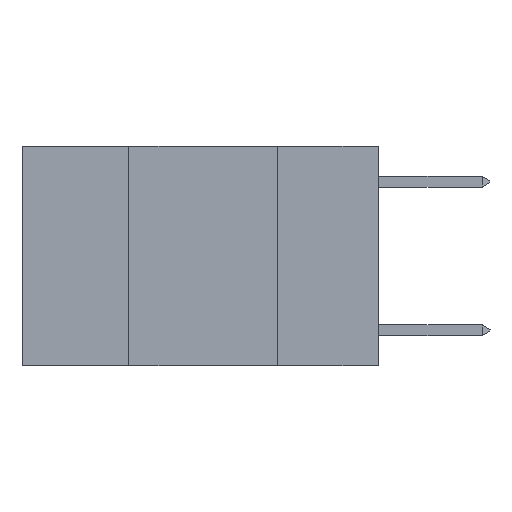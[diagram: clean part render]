
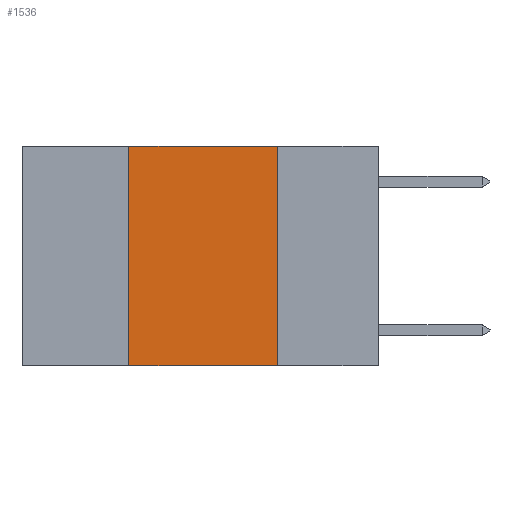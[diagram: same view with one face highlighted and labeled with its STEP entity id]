
A CAD part, left-side view. The second image highlights one B-rep face of the part: STEP entity #1536.
In plain terms, the highlighted planar face has unit normal (-1, 0, 0).
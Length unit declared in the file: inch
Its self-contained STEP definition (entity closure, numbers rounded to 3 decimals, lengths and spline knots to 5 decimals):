
#22 = CARTESIAN_POINT ( 'NONE',  ( 0., 0.17, 0. ) ) ;
#275 = EDGE_CURVE ( 'NONE', #723, #17620, #13090, .T. ) ;
#723 = VERTEX_POINT ( 'NONE', #16171 ) ;
#1536 = ADVANCED_FACE ( 'NONE', ( #12596 ), #6513, .F. ) ;
#1971 = EDGE_LOOP ( 'NONE', ( #5918, #19016, #5933, #5943 ) ) ;
#3739 = CARTESIAN_POINT ( 'NONE',  ( 0., 0.6, -0.37 ) ) ;
#4003 = VECTOR ( 'NONE', #4907, 39.37008 ) ;
#4252 = VERTEX_POINT ( 'NONE', #18036 ) ;
#4571 = CARTESIAN_POINT ( 'NONE',  ( 0., 0.17, -0.37 ) ) ;
#4907 = DIRECTION ( 'NONE',  ( 0., -1., 0. ) ) ;
#5918 = ORIENTED_EDGE ( 'NONE', *, *, #7991, .F. ) ;
#5933 = ORIENTED_EDGE ( 'NONE', *, *, #17792, .F. ) ;
#5943 = ORIENTED_EDGE ( 'NONE', *, *, #275, .T. ) ;
#6513 = PLANE ( 'NONE',  #15474 ) ;
#7655 = EDGE_CURVE ( 'NONE', #4252, #19973, #13603, .T. ) ;
#7675 = DIRECTION ( 'NONE',  ( 0., 0., -1. ) ) ;
#7991 = EDGE_CURVE ( 'NONE', #19973, #17620, #14310, .T. ) ;
#9720 = LINE ( 'NONE', #11394, #17651 ) ;
#11394 = CARTESIAN_POINT ( 'NONE',  ( 0., 0.42, 0. ) ) ;
#12596 = FACE_OUTER_BOUND ( 'NONE', #1971, .T. ) ;
#12691 = DIRECTION ( 'NONE',  ( 1., 0., 0. ) ) ;
#12811 = CARTESIAN_POINT ( 'NONE',  ( 0., 0.17, 0. ) ) ;
#13090 = LINE ( 'NONE', #3739, #4003 ) ;
#13603 = LINE ( 'NONE', #19929, #19804 ) ;
#14310 = LINE ( 'NONE', #22, #16491 ) ;
#15474 = AXIS2_PLACEMENT_3D ( 'NONE', #18820, #12691, #7675 ) ;
#16164 = DIRECTION ( 'NONE',  ( 0., 0., -1. ) ) ;
#16171 = CARTESIAN_POINT ( 'NONE',  ( 0., 0.42, -0.37 ) ) ;
#16491 = VECTOR ( 'NONE', #16164, 39.37008 ) ;
#17620 = VERTEX_POINT ( 'NONE', #4571 ) ;
#17651 = VECTOR ( 'NONE', #17725, 39.37008 ) ;
#17725 = DIRECTION ( 'NONE',  ( 0., 0., 1. ) ) ;
#17792 = EDGE_CURVE ( 'NONE', #723, #4252, #9720, .T. ) ;
#18036 = CARTESIAN_POINT ( 'NONE',  ( 0., 0.42, 0. ) ) ;
#18820 = CARTESIAN_POINT ( 'NONE',  ( 0., 0.6, 0. ) ) ;
#19016 = ORIENTED_EDGE ( 'NONE', *, *, #7655, .F. ) ;
#19713 = DIRECTION ( 'NONE',  ( 0., -1., 0. ) ) ;
#19804 = VECTOR ( 'NONE', #19713, 39.37008 ) ;
#19929 = CARTESIAN_POINT ( 'NONE',  ( 0., 0.6, 0. ) ) ;
#19973 = VERTEX_POINT ( 'NONE', #12811 ) ;
